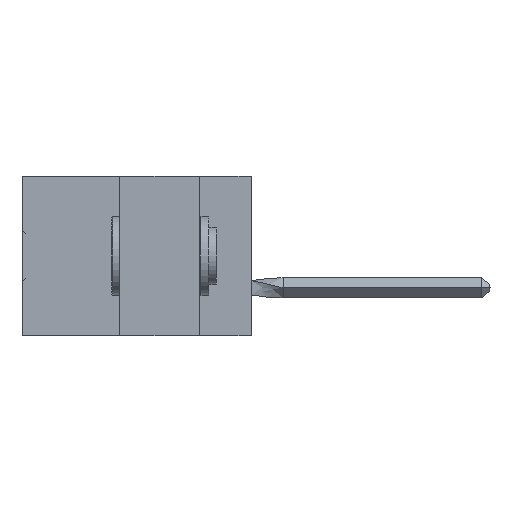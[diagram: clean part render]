
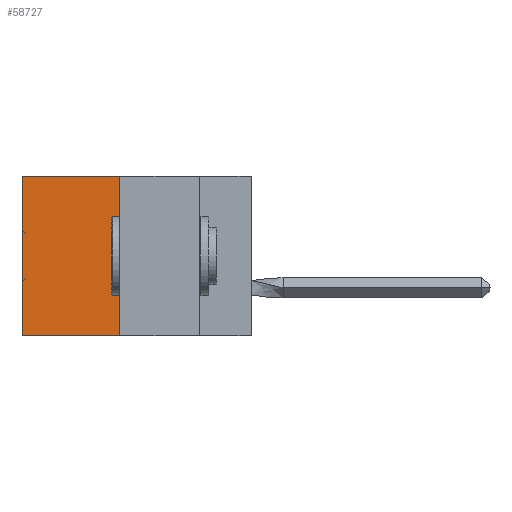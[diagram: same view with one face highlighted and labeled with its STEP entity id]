
A CAD part, left-side view. The second image highlights one B-rep face of the part: STEP entity #58727.
In plain terms, the highlighted planar face has unit normal (-1, 0, 0).
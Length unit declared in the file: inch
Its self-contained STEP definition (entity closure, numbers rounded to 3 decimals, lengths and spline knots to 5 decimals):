
#624 = CARTESIAN_POINT ( 'NONE',  ( 0.305, 0.72, 0. ) ) ;
#5477 = CARTESIAN_POINT ( 'NONE',  ( 0.305, 0.413, -0.5 ) ) ;
#5948 = VECTOR ( 'NONE', #33854, 39.37008 ) ;
#7289 = CARTESIAN_POINT ( 'NONE',  ( 0.305, 0.72, -0.5 ) ) ;
#7596 = ORIENTED_EDGE ( 'NONE', *, *, #18229, .F. ) ;
#13039 = CARTESIAN_POINT ( 'NONE',  ( 0.305, 0.413, 0. ) ) ;
#13950 = CARTESIAN_POINT ( 'NONE',  ( 0.305, 0.413, -0.5 ) ) ;
#14715 = VERTEX_POINT ( 'NONE', #31194 ) ;
#15691 = CARTESIAN_POINT ( 'NONE',  ( 0.305, 0.413, -0.5 ) ) ;
#16235 = VECTOR ( 'NONE', #17287, 39.37008 ) ;
#17287 = DIRECTION ( 'NONE',  ( 0., 1., 0. ) ) ;
#17387 = LINE ( 'NONE', #15691, #26796 ) ;
#18229 = EDGE_CURVE ( 'NONE', #44810, #14715, #17387, .T. ) ;
#18524 = VERTEX_POINT ( 'NONE', #624 ) ;
#22727 = LINE ( 'NONE', #13039, #16235 ) ;
#23056 = PLANE ( 'NONE',  #28816 ) ;
#23684 = DIRECTION ( 'NONE',  ( 1., 0., 0. ) ) ;
#25228 = DIRECTION ( 'NONE',  ( 0., 0., -1. ) ) ;
#25860 = EDGE_CURVE ( 'NONE', #44810, #18524, #22727, .T. ) ;
#26796 = VECTOR ( 'NONE', #25228, 39.37008 ) ;
#26847 = ORIENTED_EDGE ( 'NONE', *, *, #25860, .T. ) ;
#28816 = AXIS2_PLACEMENT_3D ( 'NONE', #13950, #23684, #37463 ) ;
#31194 = CARTESIAN_POINT ( 'NONE',  ( 0.305, 0.413, -0.5 ) ) ;
#33332 = ORIENTED_EDGE ( 'NONE', *, *, #36607, .T. ) ;
#33854 = DIRECTION ( 'NONE',  ( 0., 1., 0. ) ) ;
#35440 = VERTEX_POINT ( 'NONE', #59639 ) ;
#36607 = EDGE_CURVE ( 'NONE', #18524, #35440, #48735, .T. ) ;
#37463 = DIRECTION ( 'NONE',  ( 0., 0., -1. ) ) ;
#38184 = EDGE_LOOP ( 'NONE', ( #33332, #38347, #7596, #26847 ) ) ;
#38347 = ORIENTED_EDGE ( 'NONE', *, *, #58777, .F. ) ;
#39681 = DIRECTION ( 'NONE',  ( 0., 0., -1. ) ) ;
#42123 = VECTOR ( 'NONE', #39681, 39.37008 ) ;
#43288 = CARTESIAN_POINT ( 'NONE',  ( 0.305, 0.413, 0. ) ) ;
#44810 = VERTEX_POINT ( 'NONE', #43288 ) ;
#48735 = LINE ( 'NONE', #7289, #42123 ) ;
#50925 = LINE ( 'NONE', #5477, #5948 ) ;
#57500 = FACE_OUTER_BOUND ( 'NONE', #38184, .T. ) ;
#58727 = ADVANCED_FACE ( 'NONE', ( #57500 ), #23056, .F. ) ;
#58777 = EDGE_CURVE ( 'NONE', #14715, #35440, #50925, .T. ) ;
#59639 = CARTESIAN_POINT ( 'NONE',  ( 0.305, 0.72, -0.5 ) ) ;
